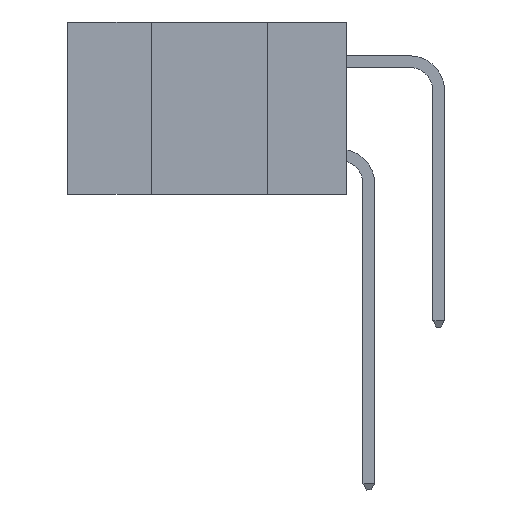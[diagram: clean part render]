
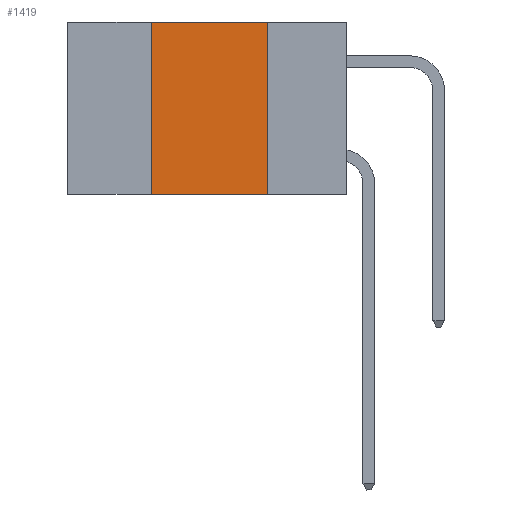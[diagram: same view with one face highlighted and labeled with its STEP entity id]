
A CAD part, left-side view. The second image highlights one B-rep face of the part: STEP entity #1419.
In plain terms, the highlighted planar face has unit normal (-1, 0, 0).
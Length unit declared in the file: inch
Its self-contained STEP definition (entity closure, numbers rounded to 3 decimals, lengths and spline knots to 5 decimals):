
#286 = DIRECTION ( 'NONE',  ( 0., 0., -1. ) ) ;
#598 = AXIS2_PLACEMENT_3D ( 'NONE', #10144, #10116, #11704 ) ;
#1111 = DIRECTION ( 'NONE',  ( 0., 0., 1. ) ) ;
#1356 = VERTEX_POINT ( 'NONE', #13003 ) ;
#1419 = ADVANCED_FACE ( 'NONE', ( #3794 ), #10069, .F. ) ;
#2366 = DIRECTION ( 'NONE',  ( 0., -1., 0. ) ) ;
#2491 = VECTOR ( 'NONE', #286, 39.37008 ) ;
#2556 = LINE ( 'NONE', #9751, #5465 ) ;
#2854 = ORIENTED_EDGE ( 'NONE', *, *, #3715, .F. ) ;
#2953 = ORIENTED_EDGE ( 'NONE', *, *, #8320, .F. ) ;
#3149 = ORIENTED_EDGE ( 'NONE', *, *, #4438, .F. ) ;
#3241 = ORIENTED_EDGE ( 'NONE', *, *, #6562, .T. ) ;
#3715 = EDGE_CURVE ( 'NONE', #11456, #1356, #7838, .T. ) ;
#3794 = FACE_OUTER_BOUND ( 'NONE', #8003, .T. ) ;
#4438 = EDGE_CURVE ( 'NONE', #10042, #11113, #6049, .T. ) ;
#5465 = VECTOR ( 'NONE', #2366, 39.37008 ) ;
#6049 = LINE ( 'NONE', #7613, #8444 ) ;
#6470 = LINE ( 'NONE', #9660, #11350 ) ;
#6562 = EDGE_CURVE ( 'NONE', #10042, #1356, #6470, .T. ) ;
#6845 = CARTESIAN_POINT ( 'NONE',  ( 0., 0.17, 0. ) ) ;
#6924 = CARTESIAN_POINT ( 'NONE',  ( 0., 0.17, 0. ) ) ;
#7613 = CARTESIAN_POINT ( 'NONE',  ( 0., 0.42, 0. ) ) ;
#7838 = LINE ( 'NONE', #6845, #2491 ) ;
#8003 = EDGE_LOOP ( 'NONE', ( #2854, #2953, #3149, #3241 ) ) ;
#8320 = EDGE_CURVE ( 'NONE', #11113, #11456, #2556, .T. ) ;
#8444 = VECTOR ( 'NONE', #1111, 39.37008 ) ;
#8621 = DIRECTION ( 'NONE',  ( 0., -1., 0. ) ) ;
#9660 = CARTESIAN_POINT ( 'NONE',  ( 0., 0.6, -0.37 ) ) ;
#9751 = CARTESIAN_POINT ( 'NONE',  ( 0., 0.6, 0. ) ) ;
#10042 = VERTEX_POINT ( 'NONE', #13555 ) ;
#10069 = PLANE ( 'NONE',  #598 ) ;
#10116 = DIRECTION ( 'NONE',  ( 1., 0., 0. ) ) ;
#10144 = CARTESIAN_POINT ( 'NONE',  ( 0., 0.6, 0. ) ) ;
#10580 = CARTESIAN_POINT ( 'NONE',  ( 0., 0.42, 0. ) ) ;
#11113 = VERTEX_POINT ( 'NONE', #10580 ) ;
#11350 = VECTOR ( 'NONE', #8621, 39.37008 ) ;
#11456 = VERTEX_POINT ( 'NONE', #6924 ) ;
#11704 = DIRECTION ( 'NONE',  ( 0., 0., -1. ) ) ;
#13003 = CARTESIAN_POINT ( 'NONE',  ( 0., 0.17, -0.37 ) ) ;
#13555 = CARTESIAN_POINT ( 'NONE',  ( 0., 0.42, -0.37 ) ) ;
